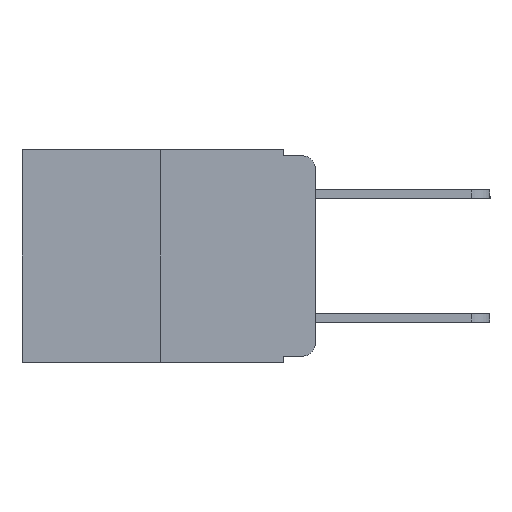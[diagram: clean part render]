
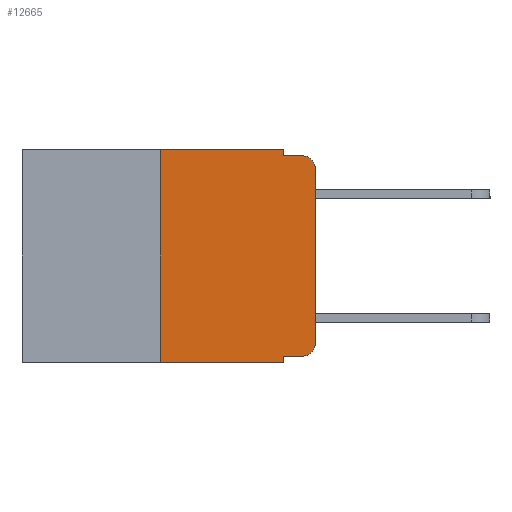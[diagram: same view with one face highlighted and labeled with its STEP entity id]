
A CAD part, left-side view. The second image highlights one B-rep face of the part: STEP entity #12665.
In plain terms, the highlighted planar face has unit normal (-1, 0, 0).
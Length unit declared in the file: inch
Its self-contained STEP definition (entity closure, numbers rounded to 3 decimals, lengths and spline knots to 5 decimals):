
#562 = LINE ( 'NONE', #10261, #18560 ) ;
#748 = ORIENTED_EDGE ( 'NONE', *, *, #10389, .T. ) ;
#950 = EDGE_CURVE ( 'NONE', #16489, #19301, #14999, .T. ) ;
#994 = LINE ( 'NONE', #9864, #19500 ) ;
#1033 = CARTESIAN_POINT ( 'NONE',  ( 0., 0.02, -0.03 ) ) ;
#1234 = CARTESIAN_POINT ( 'NONE',  ( 0., 0.051, 0. ) ) ;
#1403 = AXIS2_PLACEMENT_3D ( 'NONE', #10107, #6575, #19252 ) ;
#1453 = ORIENTED_EDGE ( 'NONE', *, *, #4711, .F. ) ;
#1748 = VECTOR ( 'NONE', #21508, 39.37008 ) ;
#2435 = VERTEX_POINT ( 'NONE', #12236 ) ;
#2492 = CARTESIAN_POINT ( 'NONE',  ( 0., 0., -0.03 ) ) ;
#2640 = ORIENTED_EDGE ( 'NONE', *, *, #5973, .F. ) ;
#2877 = CARTESIAN_POINT ( 'NONE',  ( 0., 0.051, -0.333 ) ) ;
#3877 = CARTESIAN_POINT ( 'NONE',  ( 0., 0.25, 0. ) ) ;
#4227 = EDGE_CURVE ( 'NONE', #11175, #17582, #15405, .T. ) ;
#4510 = AXIS2_PLACEMENT_3D ( 'NONE', #22437, #5041, #15677 ) ;
#4711 = EDGE_CURVE ( 'NONE', #16151, #22088, #562, .T. ) ;
#4931 = VERTEX_POINT ( 'NONE', #22200 ) ;
#5041 = DIRECTION ( 'NONE',  ( -1., 0., 0. ) ) ;
#5312 = CARTESIAN_POINT ( 'NONE',  ( 0., 0., 0. ) ) ;
#5511 = EDGE_CURVE ( 'NONE', #18867, #6311, #6891, .T. ) ;
#5874 = CARTESIAN_POINT ( 'NONE',  ( 0., 0.02, -0.333 ) ) ;
#5973 = EDGE_CURVE ( 'NONE', #2435, #4931, #15901, .T. ) ;
#6311 = VERTEX_POINT ( 'NONE', #7204 ) ;
#6575 = DIRECTION ( 'NONE',  ( 1., 0., 0. ) ) ;
#6729 = VECTOR ( 'NONE', #22742, 39.37008 ) ;
#6796 = CARTESIAN_POINT ( 'NONE',  ( 0., 0.051, -0.01 ) ) ;
#6891 = LINE ( 'NONE', #1234, #15369 ) ;
#7204 = CARTESIAN_POINT ( 'NONE',  ( 0., 0.051, -0.01 ) ) ;
#7403 = ORIENTED_EDGE ( 'NONE', *, *, #5511, .F. ) ;
#7538 = DIRECTION ( 'NONE',  ( 0., -1., 0. ) ) ;
#7775 = LINE ( 'NONE', #6796, #21609 ) ;
#8596 = EDGE_CURVE ( 'NONE', #2435, #22088, #15764, .T. ) ;
#8804 = DIRECTION ( 'NONE',  ( 0., 0., -1. ) ) ;
#9864 = CARTESIAN_POINT ( 'NONE',  ( 0., 0.051, -0.333 ) ) ;
#10107 = CARTESIAN_POINT ( 'NONE',  ( 0., 0.473, 0. ) ) ;
#10261 = CARTESIAN_POINT ( 'NONE',  ( 0., 0.051, 0. ) ) ;
#10389 = EDGE_CURVE ( 'NONE', #19301, #11175, #10599, .T. ) ;
#10424 = EDGE_LOOP ( 'NONE', ( #748, #17877, #14724, #7403, #22371, #2640, #20143, #1453, #17368, #22722 ) ) ;
#10491 = FACE_OUTER_BOUND ( 'NONE', #10424, .T. ) ;
#10508 = CARTESIAN_POINT ( 'NONE',  ( 0., 0.02, -0.01 ) ) ;
#10599 = LINE ( 'NONE', #5312, #19714 ) ;
#10652 = DIRECTION ( 'NONE',  ( 0., 0., -1. ) ) ;
#11175 = VERTEX_POINT ( 'NONE', #2492 ) ;
#11978 = LINE ( 'NONE', #12852, #13117 ) ;
#12236 = CARTESIAN_POINT ( 'NONE',  ( 0., 0.25, -0.343 ) ) ;
#12665 = ADVANCED_FACE ( 'NONE', ( #10491 ), #17434, .F. ) ;
#12852 = CARTESIAN_POINT ( 'NONE',  ( 0., 0.473, 0. ) ) ;
#13117 = VECTOR ( 'NONE', #7538, 39.37008 ) ;
#14650 = AXIS2_PLACEMENT_3D ( 'NONE', #1033, #23665, #8804 ) ;
#14724 = ORIENTED_EDGE ( 'NONE', *, *, #18623, .F. ) ;
#14954 = CARTESIAN_POINT ( 'NONE',  ( 0., 0.051, -0.343 ) ) ;
#14999 = CIRCLE ( 'NONE', #4510, 0.02 ) ;
#15369 = VECTOR ( 'NONE', #21237, 39.37008 ) ;
#15405 = CIRCLE ( 'NONE', #14650, 0.02 ) ;
#15677 = DIRECTION ( 'NONE',  ( 0., 0., -1. ) ) ;
#15689 = CARTESIAN_POINT ( 'NONE',  ( 0., 0.473, -0.343 ) ) ;
#15764 = LINE ( 'NONE', #15689, #6729 ) ;
#15839 = CARTESIAN_POINT ( 'NONE',  ( 0., 0., -0.313 ) ) ;
#15901 = LINE ( 'NONE', #3877, #1748 ) ;
#16151 = VERTEX_POINT ( 'NONE', #2877 ) ;
#16204 = DIRECTION ( 'NONE',  ( 0., 0., 1. ) ) ;
#16489 = VERTEX_POINT ( 'NONE', #5874 ) ;
#16512 = CARTESIAN_POINT ( 'NONE',  ( 0., 0.051, 0. ) ) ;
#17368 = ORIENTED_EDGE ( 'NONE', *, *, #22210, .T. ) ;
#17434 = PLANE ( 'NONE',  #1403 ) ;
#17582 = VERTEX_POINT ( 'NONE', #10508 ) ;
#17877 = ORIENTED_EDGE ( 'NONE', *, *, #4227, .T. ) ;
#18237 = EDGE_CURVE ( 'NONE', #4931, #18867, #11978, .T. ) ;
#18560 = VECTOR ( 'NONE', #10652, 39.37008 ) ;
#18623 = EDGE_CURVE ( 'NONE', #6311, #17582, #7775, .T. ) ;
#18867 = VERTEX_POINT ( 'NONE', #16512 ) ;
#19252 = DIRECTION ( 'NONE',  ( 0., 0., -1. ) ) ;
#19301 = VERTEX_POINT ( 'NONE', #15839 ) ;
#19460 = DIRECTION ( 'NONE',  ( 0., -1., 0. ) ) ;
#19500 = VECTOR ( 'NONE', #20710, 39.37008 ) ;
#19714 = VECTOR ( 'NONE', #16204, 39.37008 ) ;
#20143 = ORIENTED_EDGE ( 'NONE', *, *, #8596, .T. ) ;
#20710 = DIRECTION ( 'NONE',  ( 0., -1., 0. ) ) ;
#21237 = DIRECTION ( 'NONE',  ( 0., 0., -1. ) ) ;
#21508 = DIRECTION ( 'NONE',  ( 0., 0., 1. ) ) ;
#21609 = VECTOR ( 'NONE', #19460, 39.37008 ) ;
#22088 = VERTEX_POINT ( 'NONE', #14954 ) ;
#22200 = CARTESIAN_POINT ( 'NONE',  ( 0., 0.25, 0. ) ) ;
#22210 = EDGE_CURVE ( 'NONE', #16151, #16489, #994, .T. ) ;
#22371 = ORIENTED_EDGE ( 'NONE', *, *, #18237, .F. ) ;
#22437 = CARTESIAN_POINT ( 'NONE',  ( 0., 0.02, -0.313 ) ) ;
#22722 = ORIENTED_EDGE ( 'NONE', *, *, #950, .T. ) ;
#22742 = DIRECTION ( 'NONE',  ( 0., -1., 0. ) ) ;
#23665 = DIRECTION ( 'NONE',  ( -1., 0., 0. ) ) ;
